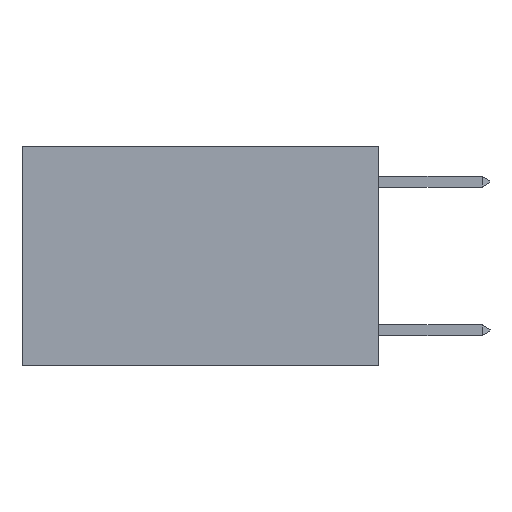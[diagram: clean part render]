
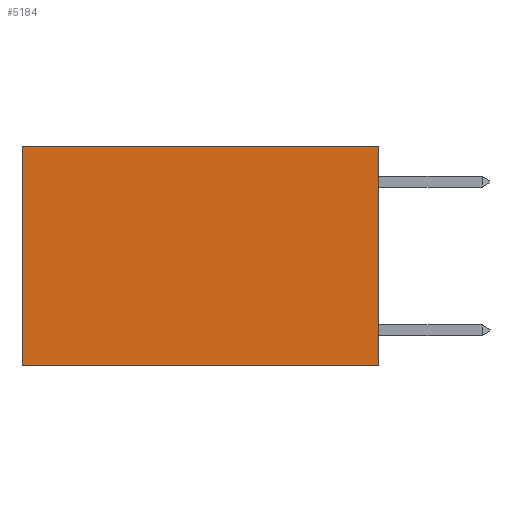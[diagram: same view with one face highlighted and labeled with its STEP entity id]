
A CAD part, left-side view. The second image highlights one B-rep face of the part: STEP entity #5184.
In plain terms, the highlighted planar face has unit normal (-1, 0, 0).
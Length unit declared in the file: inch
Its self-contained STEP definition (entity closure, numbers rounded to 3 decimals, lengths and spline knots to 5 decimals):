
#92 = VERTEX_POINT ( 'NONE', #6312 ) ;
#322 = LINE ( 'NONE', #9951, #6182 ) ;
#350 = ORIENTED_EDGE ( 'NONE', *, *, #5088, .T. ) ;
#899 = ORIENTED_EDGE ( 'NONE', *, *, #11003, .T. ) ;
#956 = CARTESIAN_POINT ( 'NONE',  ( 0.2625, 0.6, 0. ) ) ;
#991 = DIRECTION ( 'NONE',  ( 1., 0., 0. ) ) ;
#2008 = DIRECTION ( 'NONE',  ( 0., 1., 0. ) ) ;
#2420 = CARTESIAN_POINT ( 'NONE',  ( 0.2625, 0., 0. ) ) ;
#2772 = ORIENTED_EDGE ( 'NONE', *, *, #11655, .F. ) ;
#3337 = EDGE_LOOP ( 'NONE', ( #899, #5427, #2772, #350 ) ) ;
#3372 = LINE ( 'NONE', #13720, #9442 ) ;
#3978 = DIRECTION ( 'NONE',  ( 0., 1., 0. ) ) ;
#4072 = VERTEX_POINT ( 'NONE', #10397 ) ;
#4204 = CARTESIAN_POINT ( 'NONE',  ( 0.2625, 0., 0. ) ) ;
#4583 = FACE_OUTER_BOUND ( 'NONE', #3337, .T. ) ;
#4806 = DIRECTION ( 'NONE',  ( 0., 0., -1. ) ) ;
#5088 = EDGE_CURVE ( 'NONE', #14427, #8603, #3372, .T. ) ;
#5184 = ADVANCED_FACE ( 'NONE', ( #4583 ), #11352, .F. ) ;
#5303 = EDGE_CURVE ( 'NONE', #92, #4072, #11128, .T. ) ;
#5427 = ORIENTED_EDGE ( 'NONE', *, *, #5303, .F. ) ;
#5635 = VECTOR ( 'NONE', #15356, 39.37008 ) ;
#6182 = VECTOR ( 'NONE', #4806, 39.37008 ) ;
#6312 = CARTESIAN_POINT ( 'NONE',  ( 0.2625, 0., -0.37 ) ) ;
#8603 = VERTEX_POINT ( 'NONE', #956 ) ;
#9118 = CARTESIAN_POINT ( 'NONE',  ( 0.2625, 0., -0.37 ) ) ;
#9442 = VECTOR ( 'NONE', #2008, 39.37008 ) ;
#9951 = CARTESIAN_POINT ( 'NONE',  ( 0.2625, 0., 0. ) ) ;
#10334 = AXIS2_PLACEMENT_3D ( 'NONE', #2420, #991, #15476 ) ;
#10397 = CARTESIAN_POINT ( 'NONE',  ( 0.2625, 0.6, -0.37 ) ) ;
#11003 = EDGE_CURVE ( 'NONE', #8603, #4072, #15669, .T. ) ;
#11128 = LINE ( 'NONE', #9118, #14233 ) ;
#11352 = PLANE ( 'NONE',  #10334 ) ;
#11655 = EDGE_CURVE ( 'NONE', #14427, #92, #322, .T. ) ;
#13720 = CARTESIAN_POINT ( 'NONE',  ( 0.2625, 0., 0. ) ) ;
#14233 = VECTOR ( 'NONE', #3978, 39.37008 ) ;
#14427 = VERTEX_POINT ( 'NONE', #4204 ) ;
#15356 = DIRECTION ( 'NONE',  ( 0., 0., -1. ) ) ;
#15476 = DIRECTION ( 'NONE',  ( 0., 0., -1. ) ) ;
#15669 = LINE ( 'NONE', #16728, #5635 ) ;
#16728 = CARTESIAN_POINT ( 'NONE',  ( 0.2625, 0.6, 0. ) ) ;
